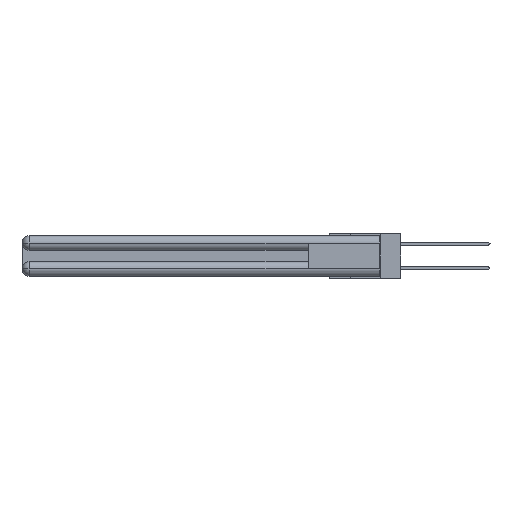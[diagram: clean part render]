
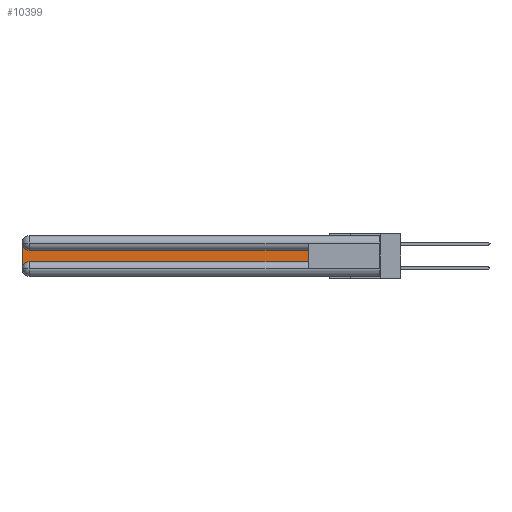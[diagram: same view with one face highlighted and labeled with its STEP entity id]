
A CAD part, left-side view. The second image highlights one B-rep face of the part: STEP entity #10399.
In plain terms, the highlighted planar face has unit normal (-1, 0, 0).
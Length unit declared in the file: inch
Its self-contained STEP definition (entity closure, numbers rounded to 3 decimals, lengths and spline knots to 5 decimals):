
#133 = ORIENTED_EDGE ( 'NONE', *, *, #11326, .T. ) ;
#239 = EDGE_LOOP ( 'NONE', ( #133, #22192, #9309, #18016, #18877, #5115 ) ) ;
#479 = DIRECTION ( 'NONE',  ( 1., 0., 0. ) ) ;
#580 = VERTEX_POINT ( 'NONE', #15060 ) ;
#1209 = DIRECTION ( 'NONE',  ( 1., 0., 0. ) ) ;
#1603 = CARTESIAN_POINT ( 'NONE',  ( 0.075, 3., -0.2175 ) ) ;
#2022 = VERTEX_POINT ( 'NONE', #17547 ) ;
#2374 = CARTESIAN_POINT ( 'NONE',  ( 0.075, 0.6, -0.1225 ) ) ;
#2395 = CARTESIAN_POINT ( 'NONE',  ( 0.075, 3., -0.1225 ) ) ;
#2541 = VERTEX_POINT ( 'NONE', #5596 ) ;
#3008 = DIRECTION ( 'NONE',  ( 0., -1., 0. ) ) ;
#4092 = CARTESIAN_POINT ( 'NONE',  ( 0.075, 0.6, -0.2175 ) ) ;
#4824 = VERTEX_POINT ( 'NONE', #10403 ) ;
#5115 = ORIENTED_EDGE ( 'NONE', *, *, #21452, .T. ) ;
#5289 = VECTOR ( 'NONE', #13486, 39.37008 ) ;
#5440 = DIRECTION ( 'NONE',  ( 0., 0., -1. ) ) ;
#5596 = CARTESIAN_POINT ( 'NONE',  ( 0.075, 3., -0.0625 ) ) ;
#6983 = DIRECTION ( 'NONE',  ( 0., 0., 1. ) ) ;
#7711 = VECTOR ( 'NONE', #3008, 39.37008 ) ;
#7769 = CARTESIAN_POINT ( 'NONE',  ( 0.075, 2.94, -0.2775 ) ) ;
#8212 = LINE ( 'NONE', #4092, #24284 ) ;
#8867 = VERTEX_POINT ( 'NONE', #2374 ) ;
#9309 = ORIENTED_EDGE ( 'NONE', *, *, #15167, .T. ) ;
#10397 = VECTOR ( 'NONE', #10624, 39.37008 ) ;
#10399 = ADVANCED_FACE ( 'NONE', ( #26215 ), #12894, .F. ) ;
#10403 = CARTESIAN_POINT ( 'NONE',  ( 0.075, 2.94, -0.2175 ) ) ;
#10624 = DIRECTION ( 'NONE',  ( 0., 0., -1. ) ) ;
#11326 = EDGE_CURVE ( 'NONE', #8867, #580, #17383, .T. ) ;
#11489 = CARTESIAN_POINT ( 'NONE',  ( 0.075, 0.6, -0.2175 ) ) ;
#11583 = AXIS2_PLACEMENT_3D ( 'NONE', #19079, #1209, #5440 ) ;
#12894 = PLANE ( 'NONE',  #24316 ) ;
#13486 = DIRECTION ( 'NONE',  ( 0., 1., 0. ) ) ;
#15060 = CARTESIAN_POINT ( 'NONE',  ( 0.075, 2.94, -0.1225 ) ) ;
#15167 = EDGE_CURVE ( 'NONE', #2541, #2022, #16798, .T. ) ;
#15949 = CIRCLE ( 'NONE', #11583, 0.06 ) ;
#16798 = LINE ( 'NONE', #1603, #10397 ) ;
#17078 = EDGE_CURVE ( 'NONE', #580, #2541, #15949, .T. ) ;
#17334 = LINE ( 'NONE', #23262, #7711 ) ;
#17383 = LINE ( 'NONE', #27158, #5289 ) ;
#17547 = CARTESIAN_POINT ( 'NONE',  ( 0.075, 3., -0.2775 ) ) ;
#18016 = ORIENTED_EDGE ( 'NONE', *, *, #28038, .T. ) ;
#18343 = DIRECTION ( 'NONE',  ( 1., 0., 0. ) ) ;
#18877 = ORIENTED_EDGE ( 'NONE', *, *, #26331, .T. ) ;
#19079 = CARTESIAN_POINT ( 'NONE',  ( 0.075, 2.94, -0.0625 ) ) ;
#19596 = AXIS2_PLACEMENT_3D ( 'NONE', #7769, #479, #21049 ) ;
#21049 = DIRECTION ( 'NONE',  ( 0., 0., -1. ) ) ;
#21452 = EDGE_CURVE ( 'NONE', #29529, #8867, #8212, .T. ) ;
#22192 = ORIENTED_EDGE ( 'NONE', *, *, #17078, .T. ) ;
#22683 = CIRCLE ( 'NONE', #19596, 0.06 ) ;
#23262 = CARTESIAN_POINT ( 'NONE',  ( 0.075, 0.6, -0.2175 ) ) ;
#24284 = VECTOR ( 'NONE', #6983, 39.37008 ) ;
#24316 = AXIS2_PLACEMENT_3D ( 'NONE', #2395, #18343, #24752 ) ;
#24752 = DIRECTION ( 'NONE',  ( 0., 0., -1. ) ) ;
#26215 = FACE_OUTER_BOUND ( 'NONE', #239, .T. ) ;
#26331 = EDGE_CURVE ( 'NONE', #4824, #29529, #17334, .T. ) ;
#27158 = CARTESIAN_POINT ( 'NONE',  ( 0.075, 0.6, -0.1225 ) ) ;
#28038 = EDGE_CURVE ( 'NONE', #2022, #4824, #22683, .T. ) ;
#29529 = VERTEX_POINT ( 'NONE', #11489 ) ;
